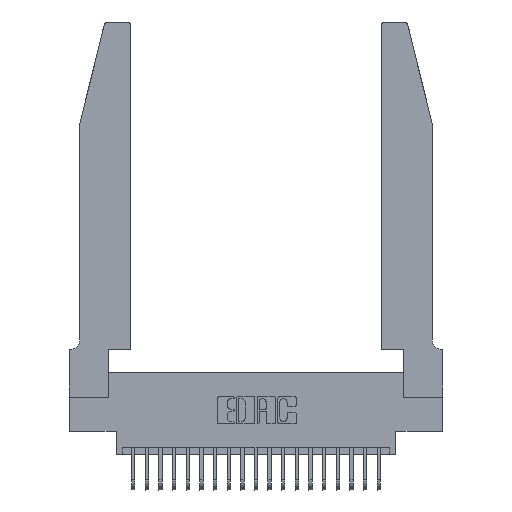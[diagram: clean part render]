
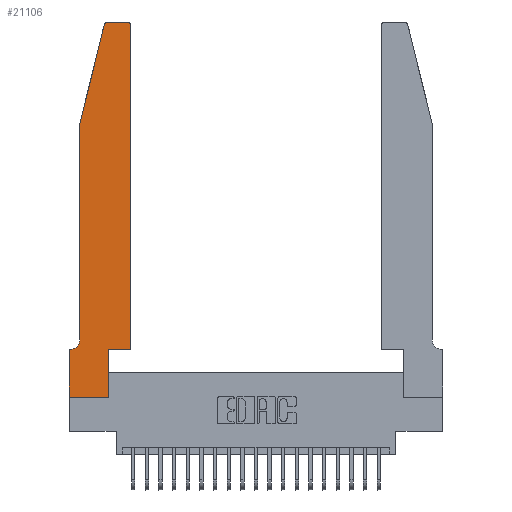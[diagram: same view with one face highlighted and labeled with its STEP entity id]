
A CAD part, top view. The second image highlights one B-rep face of the part: STEP entity #21106.
In plain terms, the highlighted planar face has unit normal (0, 0, 1).
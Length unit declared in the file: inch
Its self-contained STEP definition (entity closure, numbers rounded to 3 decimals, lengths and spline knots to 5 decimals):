
#313 = AXIS2_PLACEMENT_3D ( 'NONE', #4359, #15702, #9979 ) ;
#392 = CARTESIAN_POINT ( 'NONE',  ( 0.4505, 0.35, 0.37 ) ) ;
#398 = VECTOR ( 'NONE', #2680, 39.37008 ) ;
#820 = EDGE_LOOP ( 'NONE', ( #7979, #14226, #15224, #22773, #10345, #6191, #16035, #1952, #3393, #2869, #8036, #1948 ) ) ;
#893 = CARTESIAN_POINT ( 'NONE',  ( 0.0755, 0.35, 0.37 ) ) ;
#1175 = CARTESIAN_POINT ( 'NONE',  ( 0., 0., 0.37 ) ) ;
#1305 = CARTESIAN_POINT ( 'NONE',  ( 0.2865, 0.35, 0.37 ) ) ;
#1414 = VERTEX_POINT ( 'NONE', #24517 ) ;
#1595 = VERTEX_POINT ( 'NONE', #3783 ) ;
#1634 = VECTOR ( 'NONE', #15302, 39.37008 ) ;
#1839 = CARTESIAN_POINT ( 'NONE',  ( 0.2865, 0.35, 0.37 ) ) ;
#1948 = ORIENTED_EDGE ( 'NONE', *, *, #6227, .T. ) ;
#1952 = ORIENTED_EDGE ( 'NONE', *, *, #16834, .T. ) ;
#2203 = CIRCLE ( 'NONE', #313, 0.03 ) ;
#2375 = DIRECTION ( 'NONE',  ( -0.239, -0.971, 0. ) ) ;
#2680 = DIRECTION ( 'NONE',  ( 0., -1., 0. ) ) ;
#2869 = ORIENTED_EDGE ( 'NONE', *, *, #21311, .T. ) ;
#3393 = ORIENTED_EDGE ( 'NONE', *, *, #4428, .T. ) ;
#3783 = CARTESIAN_POINT ( 'NONE',  ( 0., 0.35, 0.37 ) ) ;
#4359 = CARTESIAN_POINT ( 'NONE',  ( 0.4205, 2.72, 0.37 ) ) ;
#4428 = EDGE_CURVE ( 'NONE', #7310, #23050, #8547, .T. ) ;
#4504 = AXIS2_PLACEMENT_3D ( 'NONE', #5141, #12765, #6889 ) ;
#5089 = DIRECTION ( 'NONE',  ( 0., 1., 0. ) ) ;
#5141 = CARTESIAN_POINT ( 'NONE',  ( 0.0055, 0.42, 0.37 ) ) ;
#5587 = VERTEX_POINT ( 'NONE', #13051 ) ;
#6191 = ORIENTED_EDGE ( 'NONE', *, *, #21414, .T. ) ;
#6227 = EDGE_CURVE ( 'NONE', #1414, #23326, #2203, .T. ) ;
#6306 = EDGE_CURVE ( 'NONE', #10067, #5587, #10818, .T. ) ;
#6889 = DIRECTION ( 'NONE',  ( -1., 0., 0. ) ) ;
#7246 = CARTESIAN_POINT ( 'NONE',  ( 0., 0.35, 0.37 ) ) ;
#7310 = VERTEX_POINT ( 'NONE', #20005 ) ;
#7979 = ORIENTED_EDGE ( 'NONE', *, *, #18376, .T. ) ;
#8036 = ORIENTED_EDGE ( 'NONE', *, *, #8575, .T. ) ;
#8447 = AXIS2_PLACEMENT_3D ( 'NONE', #23296, #17576, #19490 ) ;
#8547 = LINE ( 'NONE', #1305, #12984 ) ;
#8575 = EDGE_CURVE ( 'NONE', #17267, #1414, #14613, .T. ) ;
#8995 = CARTESIAN_POINT ( 'NONE',  ( 0.0055, 0.35, 0.37 ) ) ;
#9342 = LINE ( 'NONE', #392, #11989 ) ;
#9536 = EDGE_CURVE ( 'NONE', #5587, #18897, #19118, .T. ) ;
#9561 = VECTOR ( 'NONE', #5089, 39.37008 ) ;
#9693 = EDGE_CURVE ( 'NONE', #23425, #10067, #11504, .T. ) ;
#9979 = DIRECTION ( 'NONE',  ( 1., 0., 0. ) ) ;
#10067 = VERTEX_POINT ( 'NONE', #19182 ) ;
#10345 = ORIENTED_EDGE ( 'NONE', *, *, #9536, .T. ) ;
#10816 = DIRECTION ( 'NONE',  ( 1., 0., 0. ) ) ;
#10818 = LINE ( 'NONE', #11971, #398 ) ;
#11031 = DIRECTION ( 'NONE',  ( 0., 0., 1. ) ) ;
#11199 = VECTOR ( 'NONE', #10816, 39.37008 ) ;
#11308 = AXIS2_PLACEMENT_3D ( 'NONE', #7246, #11031, #16594 ) ;
#11504 = LINE ( 'NONE', #15630, #23460 ) ;
#11971 = CARTESIAN_POINT ( 'NONE',  ( 0.0755, 2., 0.37 ) ) ;
#11989 = VECTOR ( 'NONE', #19233, 39.37008 ) ;
#12021 = VERTEX_POINT ( 'NONE', #15609 ) ;
#12564 = VECTOR ( 'NONE', #16065, 39.37008 ) ;
#12702 = EDGE_CURVE ( 'NONE', #1595, #18709, #20940, .T. ) ;
#12765 = DIRECTION ( 'NONE',  ( 0., 0., -1. ) ) ;
#12918 = CARTESIAN_POINT ( 'NONE',  ( 0., 0., 0.37 ) ) ;
#12984 = VECTOR ( 'NONE', #20897, 39.37008 ) ;
#13051 = CARTESIAN_POINT ( 'NONE',  ( 0.0755, 0.42, 0.37 ) ) ;
#13833 = CARTESIAN_POINT ( 'NONE',  ( 0.4205, 2.75, 0.37 ) ) ;
#14090 = VECTOR ( 'NONE', #16891, 39.37008 ) ;
#14226 = ORIENTED_EDGE ( 'NONE', *, *, #19885, .T. ) ;
#14613 = LINE ( 'NONE', #20105, #9561 ) ;
#14864 = PLANE ( 'NONE',  #11308 ) ;
#15224 = ORIENTED_EDGE ( 'NONE', *, *, #9693, .T. ) ;
#15302 = DIRECTION ( 'NONE',  ( -1., 0., 0. ) ) ;
#15609 = CARTESIAN_POINT ( 'NONE',  ( 0.284, 2.75, 0.37 ) ) ;
#15630 = CARTESIAN_POINT ( 'NONE',  ( 0.0755, 2., 0.37 ) ) ;
#15702 = DIRECTION ( 'NONE',  ( 0., 0., 1. ) ) ;
#15844 = FACE_OUTER_BOUND ( 'NONE', #820, .T. ) ;
#16035 = ORIENTED_EDGE ( 'NONE', *, *, #12702, .T. ) ;
#16065 = DIRECTION ( 'NONE',  ( -1., 0., 0. ) ) ;
#16594 = DIRECTION ( 'NONE',  ( 1., 0., 0. ) ) ;
#16834 = EDGE_CURVE ( 'NONE', #18709, #7310, #17109, .T. ) ;
#16891 = DIRECTION ( 'NONE',  ( 0., -1., 0. ) ) ;
#17109 = LINE ( 'NONE', #18451, #11199 ) ;
#17112 = CARTESIAN_POINT ( 'NONE',  ( 0.2605, 2.75, 0.37 ) ) ;
#17267 = VERTEX_POINT ( 'NONE', #17503 ) ;
#17343 = LINE ( 'NONE', #17112, #1634 ) ;
#17503 = CARTESIAN_POINT ( 'NONE',  ( 0.4505, 0.35, 0.37 ) ) ;
#17576 = DIRECTION ( 'NONE',  ( 0., 0., 1. ) ) ;
#17603 = LINE ( 'NONE', #893, #12564 ) ;
#17893 = CARTESIAN_POINT ( 'NONE',  ( 0.25487, 2.72718, 0.37 ) ) ;
#18376 = EDGE_CURVE ( 'NONE', #23326, #12021, #17343, .T. ) ;
#18451 = CARTESIAN_POINT ( 'NONE',  ( 0., 0., 0.37 ) ) ;
#18636 = CIRCLE ( 'NONE', #8447, 0.03 ) ;
#18709 = VERTEX_POINT ( 'NONE', #1175 ) ;
#18897 = VERTEX_POINT ( 'NONE', #8995 ) ;
#19118 = CIRCLE ( 'NONE', #4504, 0.07 ) ;
#19182 = CARTESIAN_POINT ( 'NONE',  ( 0.0755, 2., 0.37 ) ) ;
#19233 = DIRECTION ( 'NONE',  ( 1., 0., 0. ) ) ;
#19490 = DIRECTION ( 'NONE',  ( 1., 0., 0. ) ) ;
#19885 = EDGE_CURVE ( 'NONE', #12021, #23425, #18636, .T. ) ;
#20005 = CARTESIAN_POINT ( 'NONE',  ( 0.2865, 0., 0.37 ) ) ;
#20105 = CARTESIAN_POINT ( 'NONE',  ( 0.4505, 0.35, 0.37 ) ) ;
#20897 = DIRECTION ( 'NONE',  ( 0., 1., 0. ) ) ;
#20940 = LINE ( 'NONE', #12918, #14090 ) ;
#21106 = ADVANCED_FACE ( 'NONE', ( #15844 ), #14864, .T. ) ;
#21311 = EDGE_CURVE ( 'NONE', #23050, #17267, #9342, .T. ) ;
#21414 = EDGE_CURVE ( 'NONE', #18897, #1595, #17603, .T. ) ;
#22773 = ORIENTED_EDGE ( 'NONE', *, *, #6306, .T. ) ;
#23050 = VERTEX_POINT ( 'NONE', #1839 ) ;
#23296 = CARTESIAN_POINT ( 'NONE',  ( 0.284, 2.72, 0.37 ) ) ;
#23326 = VERTEX_POINT ( 'NONE', #13833 ) ;
#23425 = VERTEX_POINT ( 'NONE', #17893 ) ;
#23460 = VECTOR ( 'NONE', #2375, 39.37008 ) ;
#24517 = CARTESIAN_POINT ( 'NONE',  ( 0.4505, 2.72, 0.37 ) ) ;
